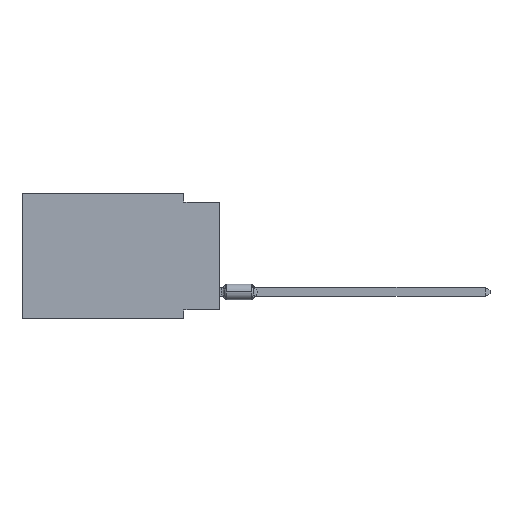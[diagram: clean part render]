
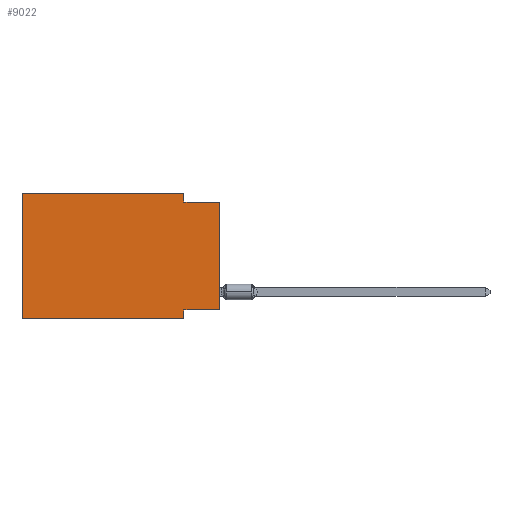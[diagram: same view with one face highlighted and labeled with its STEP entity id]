
A CAD part, left-side view. The second image highlights one B-rep face of the part: STEP entity #9022.
In plain terms, the highlighted planar face has unit normal (-1, 0, 0).
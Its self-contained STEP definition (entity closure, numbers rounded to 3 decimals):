
#86 = LINE ( 'NONE', #1303, #3419 ) ;
#98 = VERTEX_POINT ( 'NONE', #5422 ) ;
#400 = CARTESIAN_POINT ( 'NONE',  ( 0., 2.54, 0. ) ) ;
#453 = DIRECTION ( 'NONE',  ( 0., 0., 1. ) ) ;
#672 = DIRECTION ( 'NONE',  ( 0., -1., 0. ) ) ;
#867 = ORIENTED_EDGE ( 'NONE', *, *, #9898, .F. ) ;
#899 = EDGE_CURVE ( 'NONE', #1367, #9554, #6054, .T. ) ;
#1095 = EDGE_CURVE ( 'NONE', #4839, #11207, #2225, .T. ) ;
#1201 = LINE ( 'NONE', #3404, #9714 ) ;
#1213 = VECTOR ( 'NONE', #6928, 1000. ) ;
#1303 = CARTESIAN_POINT ( 'NONE',  ( 0., 0., -8.255 ) ) ;
#1367 = VERTEX_POINT ( 'NONE', #12093 ) ;
#1474 = CARTESIAN_POINT ( 'NONE',  ( 0., 13.97, 0. ) ) ;
#1810 = VECTOR ( 'NONE', #4444, 1000. ) ;
#1898 = CARTESIAN_POINT ( 'NONE',  ( 0., 2.54, -8.89 ) ) ;
#2142 = DIRECTION ( 'NONE',  ( 0., -1., 0. ) ) ;
#2225 = LINE ( 'NONE', #11556, #3588 ) ;
#2919 = ORIENTED_EDGE ( 'NONE', *, *, #1095, .T. ) ;
#2976 = CARTESIAN_POINT ( 'NONE',  ( 0., 2.54, -8.89 ) ) ;
#3404 = CARTESIAN_POINT ( 'NONE',  ( 0., 13.97, -8.89 ) ) ;
#3419 = VECTOR ( 'NONE', #6467, 1000. ) ;
#3437 = EDGE_CURVE ( 'NONE', #4380, #9554, #1201, .T. ) ;
#3438 = CARTESIAN_POINT ( 'NONE',  ( 0., 13.97, -8.89 ) ) ;
#3588 = VECTOR ( 'NONE', #4235, 1000. ) ;
#3613 = ORIENTED_EDGE ( 'NONE', *, *, #899, .F. ) ;
#4235 = DIRECTION ( 'NONE',  ( 0., 0., 1. ) ) ;
#4333 = EDGE_CURVE ( 'NONE', #98, #8562, #7742, .T. ) ;
#4380 = VERTEX_POINT ( 'NONE', #3438 ) ;
#4444 = DIRECTION ( 'NONE',  ( 0., -1., 0. ) ) ;
#4568 = CARTESIAN_POINT ( 'NONE',  ( 0., 0., -0.635 ) ) ;
#4641 = CARTESIAN_POINT ( 'NONE',  ( 0., 13.97, 0. ) ) ;
#4839 = VERTEX_POINT ( 'NONE', #10063 ) ;
#5257 = ORIENTED_EDGE ( 'NONE', *, *, #8041, .F. ) ;
#5422 = CARTESIAN_POINT ( 'NONE',  ( 0., 13.97, 0. ) ) ;
#5744 = PLANE ( 'NONE',  #12565 ) ;
#5812 = VECTOR ( 'NONE', #453, 1000. ) ;
#5882 = DIRECTION ( 'NONE',  ( 0., 0., -1. ) ) ;
#6054 = LINE ( 'NONE', #1898, #1213 ) ;
#6294 = EDGE_LOOP ( 'NONE', ( #2919, #867, #9223, #11016, #10963, #7835, #3613, #5257 ) ) ;
#6467 = DIRECTION ( 'NONE',  ( 0., 1., 0. ) ) ;
#6685 = FACE_OUTER_BOUND ( 'NONE', #6294, .T. ) ;
#6802 = EDGE_CURVE ( 'NONE', #8562, #9800, #12635, .T. ) ;
#6928 = DIRECTION ( 'NONE',  ( 0., 0., -1. ) ) ;
#7742 = LINE ( 'NONE', #4641, #1810 ) ;
#7763 = DIRECTION ( 'NONE',  ( 1., 0., 0. ) ) ;
#7835 = ORIENTED_EDGE ( 'NONE', *, *, #3437, .T. ) ;
#8041 = EDGE_CURVE ( 'NONE', #4839, #1367, #86, .T. ) ;
#8533 = DIRECTION ( 'NONE',  ( 0., 0., -1. ) ) ;
#8562 = VERTEX_POINT ( 'NONE', #8607 ) ;
#8607 = CARTESIAN_POINT ( 'NONE',  ( 0., 2.54, 0. ) ) ;
#9022 = ADVANCED_FACE ( 'NONE', ( #6685 ), #5744, .F. ) ;
#9223 = ORIENTED_EDGE ( 'NONE', *, *, #6802, .F. ) ;
#9551 = CARTESIAN_POINT ( 'NONE',  ( 0., 2.54, -0.635 ) ) ;
#9554 = VERTEX_POINT ( 'NONE', #2976 ) ;
#9714 = VECTOR ( 'NONE', #2142, 1000. ) ;
#9800 = VERTEX_POINT ( 'NONE', #9551 ) ;
#9898 = EDGE_CURVE ( 'NONE', #9800, #11207, #12708, .T. ) ;
#10063 = CARTESIAN_POINT ( 'NONE',  ( 0., 0., -8.255 ) ) ;
#10930 = VECTOR ( 'NONE', #8533, 1000. ) ;
#10963 = ORIENTED_EDGE ( 'NONE', *, *, #12134, .F. ) ;
#11016 = ORIENTED_EDGE ( 'NONE', *, *, #4333, .F. ) ;
#11207 = VERTEX_POINT ( 'NONE', #11331 ) ;
#11331 = CARTESIAN_POINT ( 'NONE',  ( 0., 0., -0.635 ) ) ;
#11556 = CARTESIAN_POINT ( 'NONE',  ( 0., 0., 0. ) ) ;
#12093 = CARTESIAN_POINT ( 'NONE',  ( 0., 2.54, -8.255 ) ) ;
#12134 = EDGE_CURVE ( 'NONE', #4380, #98, #12689, .T. ) ;
#12565 = AXIS2_PLACEMENT_3D ( 'NONE', #12872, #7763, #5882 ) ;
#12635 = LINE ( 'NONE', #400, #10930 ) ;
#12689 = LINE ( 'NONE', #1474, #5812 ) ;
#12708 = LINE ( 'NONE', #4568, #12796 ) ;
#12796 = VECTOR ( 'NONE', #672, 1000. ) ;
#12872 = CARTESIAN_POINT ( 'NONE',  ( 0., 13.97, 0. ) ) ;
